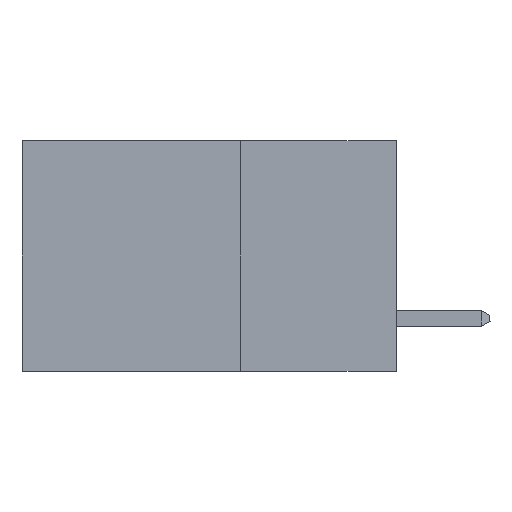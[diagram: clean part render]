
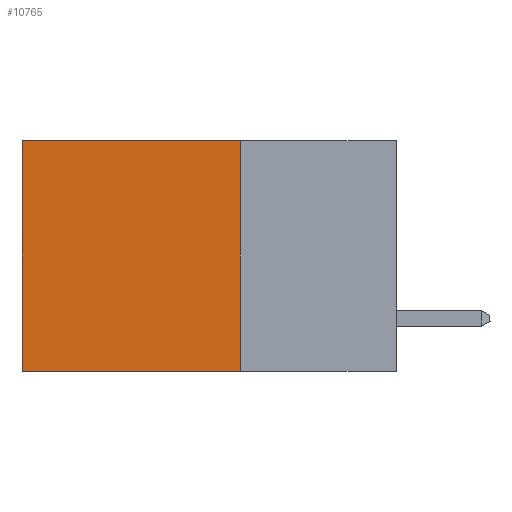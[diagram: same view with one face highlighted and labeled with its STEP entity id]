
A CAD part, left-side view. The second image highlights one B-rep face of the part: STEP entity #10765.
In plain terms, the highlighted planar face has unit normal (-1, 0, 0).
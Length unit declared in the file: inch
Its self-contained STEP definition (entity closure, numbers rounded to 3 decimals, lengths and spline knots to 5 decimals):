
#296 = VERTEX_POINT ( 'NONE', #8243 ) ;
#462 = DIRECTION ( 'NONE',  ( 0., 0., -1. ) ) ;
#677 = VERTEX_POINT ( 'NONE', #1186 ) ;
#784 = EDGE_CURVE ( 'NONE', #296, #9893, #10998, .T. ) ;
#993 = DIRECTION ( 'NONE',  ( 0., 0., -1. ) ) ;
#1186 = CARTESIAN_POINT ( 'NONE',  ( 0.298, 0.6, 0. ) ) ;
#2096 = LINE ( 'NONE', #12261, #3661 ) ;
#2973 = ORIENTED_EDGE ( 'NONE', *, *, #784, .F. ) ;
#3259 = CARTESIAN_POINT ( 'NONE',  ( 0.298, 0.6, -0.37 ) ) ;
#3661 = VECTOR ( 'NONE', #6886, 39.37008 ) ;
#4368 = DIRECTION ( 'NONE',  ( 1., 0., 0. ) ) ;
#4766 = CARTESIAN_POINT ( 'NONE',  ( 0.298, 0.25, -0.37 ) ) ;
#4770 = FACE_OUTER_BOUND ( 'NONE', #11527, .T. ) ;
#5115 = LINE ( 'NONE', #10027, #13385 ) ;
#5366 = DIRECTION ( 'NONE',  ( 0., 0., -1. ) ) ;
#6529 = ORIENTED_EDGE ( 'NONE', *, *, #10239, .T. ) ;
#6598 = ORIENTED_EDGE ( 'NONE', *, *, #10707, .F. ) ;
#6791 = LINE ( 'NONE', #9748, #13702 ) ;
#6886 = DIRECTION ( 'NONE',  ( 0., 1., 0. ) ) ;
#6896 = DIRECTION ( 'NONE',  ( 0., 1., 0. ) ) ;
#7153 = ORIENTED_EDGE ( 'NONE', *, *, #13960, .T. ) ;
#8243 = CARTESIAN_POINT ( 'NONE',  ( 0.298, 0.25, -0.37 ) ) ;
#8256 = CARTESIAN_POINT ( 'NONE',  ( 0.298, 0.25, 0. ) ) ;
#8476 = VECTOR ( 'NONE', #6896, 39.37008 ) ;
#9748 = CARTESIAN_POINT ( 'NONE',  ( 0.298, 0.25, 0. ) ) ;
#9893 = VERTEX_POINT ( 'NONE', #3259 ) ;
#10027 = CARTESIAN_POINT ( 'NONE',  ( 0.298, 0.6, 0. ) ) ;
#10239 = EDGE_CURVE ( 'NONE', #677, #9893, #5115, .T. ) ;
#10278 = AXIS2_PLACEMENT_3D ( 'NONE', #11815, #4368, #5366 ) ;
#10641 = VERTEX_POINT ( 'NONE', #8256 ) ;
#10707 = EDGE_CURVE ( 'NONE', #10641, #296, #6791, .T. ) ;
#10765 = ADVANCED_FACE ( 'NONE', ( #4770 ), #11916, .F. ) ;
#10998 = LINE ( 'NONE', #4766, #8476 ) ;
#11527 = EDGE_LOOP ( 'NONE', ( #6529, #2973, #6598, #7153 ) ) ;
#11815 = CARTESIAN_POINT ( 'NONE',  ( 0.298, 0.25, 0. ) ) ;
#11916 = PLANE ( 'NONE',  #10278 ) ;
#12261 = CARTESIAN_POINT ( 'NONE',  ( 0.298, 0.25, 0. ) ) ;
#13385 = VECTOR ( 'NONE', #462, 39.37008 ) ;
#13702 = VECTOR ( 'NONE', #993, 39.37008 ) ;
#13960 = EDGE_CURVE ( 'NONE', #10641, #677, #2096, .T. ) ;
